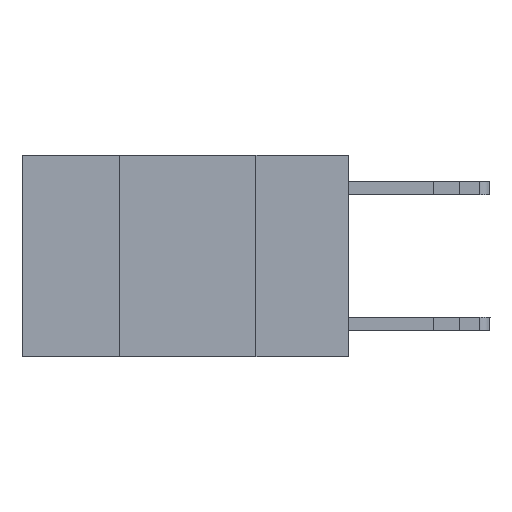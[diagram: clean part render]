
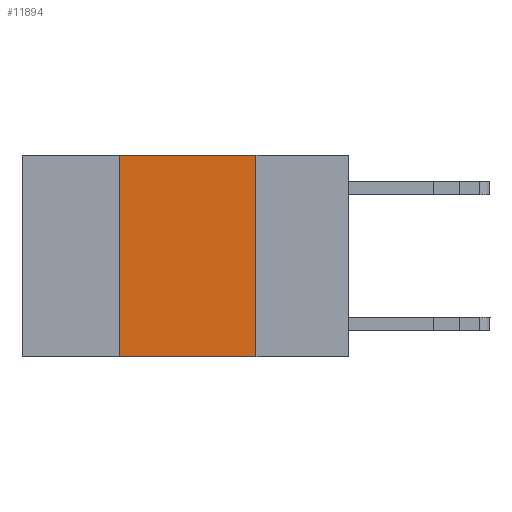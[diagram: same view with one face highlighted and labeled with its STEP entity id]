
A CAD part, left-side view. The second image highlights one B-rep face of the part: STEP entity #11894.
In plain terms, the highlighted planar face has unit normal (-1, 0, 0).
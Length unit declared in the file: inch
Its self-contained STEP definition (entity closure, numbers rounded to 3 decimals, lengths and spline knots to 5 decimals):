
#72 = PLANE ( 'NONE',  #9474 ) ;
#388 = VERTEX_POINT ( 'NONE', #12718 ) ;
#858 = CARTESIAN_POINT ( 'NONE',  ( 0., 0.17, -0.37 ) ) ;
#967 = LINE ( 'NONE', #10337, #3076 ) ;
#1115 = DIRECTION ( 'NONE',  ( 0., 0., -1. ) ) ;
#1174 = VECTOR ( 'NONE', #6113, 39.37008 ) ;
#1560 = ORIENTED_EDGE ( 'NONE', *, *, #6086, .F. ) ;
#1823 = LINE ( 'NONE', #11961, #1174 ) ;
#2332 = EDGE_CURVE ( 'NONE', #6906, #388, #4788, .T. ) ;
#2651 = VERTEX_POINT ( 'NONE', #858 ) ;
#2847 = VERTEX_POINT ( 'NONE', #11123 ) ;
#3076 = VECTOR ( 'NONE', #11289, 39.37008 ) ;
#3149 = CARTESIAN_POINT ( 'NONE',  ( 0., 0.6, 0. ) ) ;
#4284 = CARTESIAN_POINT ( 'NONE',  ( 0., 0.42, 0. ) ) ;
#4788 = LINE ( 'NONE', #4284, #7466 ) ;
#5614 = CARTESIAN_POINT ( 'NONE',  ( 0., 0.17, 0. ) ) ;
#6086 = EDGE_CURVE ( 'NONE', #388, #2847, #1823, .T. ) ;
#6113 = DIRECTION ( 'NONE',  ( 0., -1., 0. ) ) ;
#6330 = DIRECTION ( 'NONE',  ( 0., 0., 1. ) ) ;
#6842 = EDGE_CURVE ( 'NONE', #2847, #2651, #10969, .T. ) ;
#6906 = VERTEX_POINT ( 'NONE', #11621 ) ;
#6934 = ORIENTED_EDGE ( 'NONE', *, *, #2332, .F. ) ;
#7186 = DIRECTION ( 'NONE',  ( 1., 0., 0. ) ) ;
#7293 = EDGE_CURVE ( 'NONE', #6906, #2651, #967, .T. ) ;
#7466 = VECTOR ( 'NONE', #6330, 39.37008 ) ;
#8404 = VECTOR ( 'NONE', #9626, 39.37008 ) ;
#8564 = FACE_OUTER_BOUND ( 'NONE', #12496, .T. ) ;
#9260 = ORIENTED_EDGE ( 'NONE', *, *, #6842, .F. ) ;
#9474 = AXIS2_PLACEMENT_3D ( 'NONE', #3149, #7186, #1115 ) ;
#9626 = DIRECTION ( 'NONE',  ( 0., 0., -1. ) ) ;
#10337 = CARTESIAN_POINT ( 'NONE',  ( 0., 0.6, -0.37 ) ) ;
#10969 = LINE ( 'NONE', #5614, #8404 ) ;
#11123 = CARTESIAN_POINT ( 'NONE',  ( 0., 0.17, 0. ) ) ;
#11289 = DIRECTION ( 'NONE',  ( 0., -1., 0. ) ) ;
#11621 = CARTESIAN_POINT ( 'NONE',  ( 0., 0.42, -0.37 ) ) ;
#11894 = ADVANCED_FACE ( 'NONE', ( #8564 ), #72, .F. ) ;
#11961 = CARTESIAN_POINT ( 'NONE',  ( 0., 0.6, 0. ) ) ;
#12087 = ORIENTED_EDGE ( 'NONE', *, *, #7293, .T. ) ;
#12496 = EDGE_LOOP ( 'NONE', ( #9260, #1560, #6934, #12087 ) ) ;
#12718 = CARTESIAN_POINT ( 'NONE',  ( 0., 0.42, 0. ) ) ;
